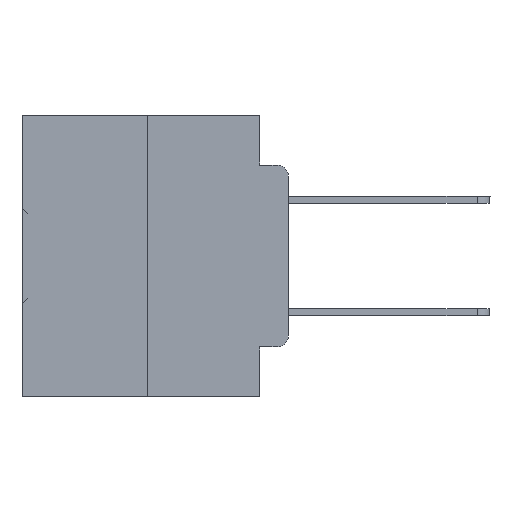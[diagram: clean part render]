
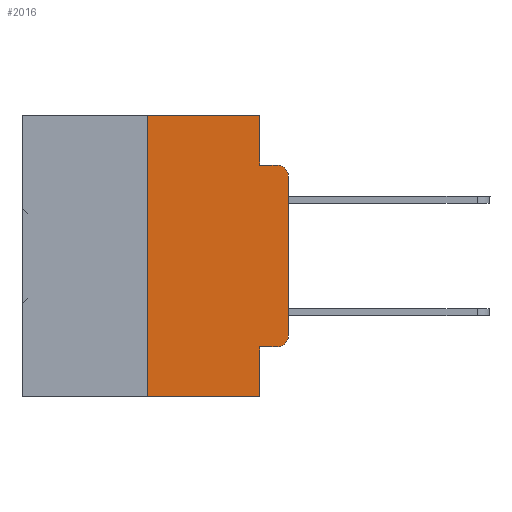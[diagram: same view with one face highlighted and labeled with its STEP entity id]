
A CAD part, left-side view. The second image highlights one B-rep face of the part: STEP entity #2016.
In plain terms, the highlighted planar face has unit normal (-1, 0, 0).
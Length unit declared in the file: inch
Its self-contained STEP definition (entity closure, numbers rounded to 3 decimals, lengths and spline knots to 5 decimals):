
#775 = ORIENTED_EDGE ( 'NONE', *, *, #19241, .F. ) ;
#872 = ORIENTED_EDGE ( 'NONE', *, *, #10711, .T. ) ;
#1531 = DIRECTION ( 'NONE',  ( 0., 0., -1. ) ) ;
#1588 = EDGE_CURVE ( 'NONE', #5838, #5229, #24735, .T. ) ;
#1623 = CARTESIAN_POINT ( 'NONE',  ( 0., 0.473, 0. ) ) ;
#2016 = ADVANCED_FACE ( 'NONE', ( #19186 ), #16284, .F. ) ;
#2621 = DIRECTION ( 'NONE',  ( -1., 0., 0. ) ) ;
#2689 = EDGE_CURVE ( 'NONE', #14761, #17330, #20386, .T. ) ;
#3755 = VECTOR ( 'NONE', #17208, 39.37008 ) ;
#4892 = CIRCLE ( 'NONE', #26691, 0.02 ) ;
#5180 = EDGE_CURVE ( 'NONE', #10948, #13971, #28652, .T. ) ;
#5229 = VERTEX_POINT ( 'NONE', #23002 ) ;
#5609 = CARTESIAN_POINT ( 'NONE',  ( 0., 0., -0.1085 ) ) ;
#5838 = VERTEX_POINT ( 'NONE', #5609 ) ;
#5850 = CARTESIAN_POINT ( 'NONE',  ( 0., 0.051, 0. ) ) ;
#5980 = ORIENTED_EDGE ( 'NONE', *, *, #2689, .T. ) ;
#6275 = CARTESIAN_POINT ( 'NONE',  ( 0., 0.051, -0.5 ) ) ;
#7393 = DIRECTION ( 'NONE',  ( 0., -1., 0. ) ) ;
#7593 = DIRECTION ( 'NONE',  ( -1., 0., 0. ) ) ;
#8787 = LINE ( 'NONE', #5850, #22685 ) ;
#8987 = VERTEX_POINT ( 'NONE', #18876 ) ;
#9204 = VECTOR ( 'NONE', #14694, 39.37008 ) ;
#9381 = VECTOR ( 'NONE', #22218, 39.37008 ) ;
#9499 = VECTOR ( 'NONE', #37057, 39.37008 ) ;
#10334 = CARTESIAN_POINT ( 'NONE',  ( 0., 0.25, 0. ) ) ;
#10440 = CARTESIAN_POINT ( 'NONE',  ( 0., 0., 0. ) ) ;
#10677 = CARTESIAN_POINT ( 'NONE',  ( 0., 0.051, -0.4115 ) ) ;
#10711 = EDGE_CURVE ( 'NONE', #17330, #17273, #4892, .T. ) ;
#10840 = VERTEX_POINT ( 'NONE', #6275 ) ;
#10948 = VERTEX_POINT ( 'NONE', #18112 ) ;
#11002 = DIRECTION ( 'NONE',  ( 0., 0., -1. ) ) ;
#12503 = EDGE_CURVE ( 'NONE', #8987, #10840, #34456, .T. ) ;
#13722 = DIRECTION ( 'NONE',  ( 1., 0., 0. ) ) ;
#13971 = VERTEX_POINT ( 'NONE', #32505 ) ;
#14375 = DIRECTION ( 'NONE',  ( 0., -1., 0. ) ) ;
#14694 = DIRECTION ( 'NONE',  ( 0., 0., -1. ) ) ;
#14761 = VERTEX_POINT ( 'NONE', #17719 ) ;
#16184 = CARTESIAN_POINT ( 'NONE',  ( 0., 0.02, -0.1085 ) ) ;
#16284 = PLANE ( 'NONE',  #26331 ) ;
#17129 = ORIENTED_EDGE ( 'NONE', *, *, #20358, .T. ) ;
#17208 = DIRECTION ( 'NONE',  ( 0., -1., 0. ) ) ;
#17273 = VERTEX_POINT ( 'NONE', #22853 ) ;
#17330 = VERTEX_POINT ( 'NONE', #36420 ) ;
#17430 = CARTESIAN_POINT ( 'NONE',  ( 0., 0.051, 0. ) ) ;
#17719 = CARTESIAN_POINT ( 'NONE',  ( 0., 0.051, -0.4115 ) ) ;
#18112 = CARTESIAN_POINT ( 'NONE',  ( 0., 0.25, 0. ) ) ;
#18542 = EDGE_CURVE ( 'NONE', #27871, #5229, #34374, .T. ) ;
#18876 = CARTESIAN_POINT ( 'NONE',  ( 0., 0.25, -0.5 ) ) ;
#19186 = FACE_OUTER_BOUND ( 'NONE', #29985, .T. ) ;
#19216 = LINE ( 'NONE', #10440, #31134 ) ;
#19241 = EDGE_CURVE ( 'NONE', #8987, #10948, #33529, .T. ) ;
#19385 = DIRECTION ( 'NONE',  ( 0., 0., -1. ) ) ;
#19622 = ORIENTED_EDGE ( 'NONE', *, *, #18542, .F. ) ;
#20107 = VECTOR ( 'NONE', #14375, 39.37008 ) ;
#20358 = EDGE_CURVE ( 'NONE', #17273, #5838, #19216, .T. ) ;
#20386 = LINE ( 'NONE', #10677, #20107 ) ;
#20651 = DIRECTION ( 'NONE',  ( 0., 0., -1. ) ) ;
#20857 = ORIENTED_EDGE ( 'NONE', *, *, #5180, .F. ) ;
#20935 = VECTOR ( 'NONE', #7393, 39.37008 ) ;
#22218 = DIRECTION ( 'NONE',  ( 0., 0., 1. ) ) ;
#22329 = DIRECTION ( 'NONE',  ( 0., 0., 1. ) ) ;
#22430 = CARTESIAN_POINT ( 'NONE',  ( 0., 0.473, 0. ) ) ;
#22685 = VECTOR ( 'NONE', #20651, 39.37008 ) ;
#22853 = CARTESIAN_POINT ( 'NONE',  ( 0., 0., -0.3915 ) ) ;
#23002 = CARTESIAN_POINT ( 'NONE',  ( 0., 0.02, -0.0885 ) ) ;
#23088 = CARTESIAN_POINT ( 'NONE',  ( 0., 0.02, -0.3915 ) ) ;
#23169 = ORIENTED_EDGE ( 'NONE', *, *, #1588, .T. ) ;
#24735 = CIRCLE ( 'NONE', #29709, 0.02 ) ;
#25093 = ORIENTED_EDGE ( 'NONE', *, *, #31367, .F. ) ;
#26331 = AXIS2_PLACEMENT_3D ( 'NONE', #1623, #13722, #19385 ) ;
#26691 = AXIS2_PLACEMENT_3D ( 'NONE', #23088, #2621, #11002 ) ;
#27871 = VERTEX_POINT ( 'NONE', #29568 ) ;
#28652 = LINE ( 'NONE', #22430, #9499 ) ;
#28717 = LINE ( 'NONE', #17430, #9204 ) ;
#28768 = ORIENTED_EDGE ( 'NONE', *, *, #12503, .T. ) ;
#29568 = CARTESIAN_POINT ( 'NONE',  ( 0., 0.051, -0.0885 ) ) ;
#29709 = AXIS2_PLACEMENT_3D ( 'NONE', #16184, #7593, #1531 ) ;
#29985 = EDGE_LOOP ( 'NONE', ( #17129, #23169, #19622, #25093, #20857, #775, #28768, #34303, #5980, #872 ) ) ;
#31134 = VECTOR ( 'NONE', #22329, 39.37008 ) ;
#31367 = EDGE_CURVE ( 'NONE', #13971, #27871, #28717, .T. ) ;
#31921 = CARTESIAN_POINT ( 'NONE',  ( 0., 0.473, -0.5 ) ) ;
#32505 = CARTESIAN_POINT ( 'NONE',  ( 0., 0.051, 0. ) ) ;
#33529 = LINE ( 'NONE', #10334, #9381 ) ;
#34303 = ORIENTED_EDGE ( 'NONE', *, *, #35265, .F. ) ;
#34374 = LINE ( 'NONE', #37315, #3755 ) ;
#34456 = LINE ( 'NONE', #31921, #20935 ) ;
#35265 = EDGE_CURVE ( 'NONE', #14761, #10840, #8787, .T. ) ;
#36420 = CARTESIAN_POINT ( 'NONE',  ( 0., 0.02, -0.4115 ) ) ;
#37057 = DIRECTION ( 'NONE',  ( 0., -1., 0. ) ) ;
#37315 = CARTESIAN_POINT ( 'NONE',  ( 0., 0.051, -0.0885 ) ) ;
